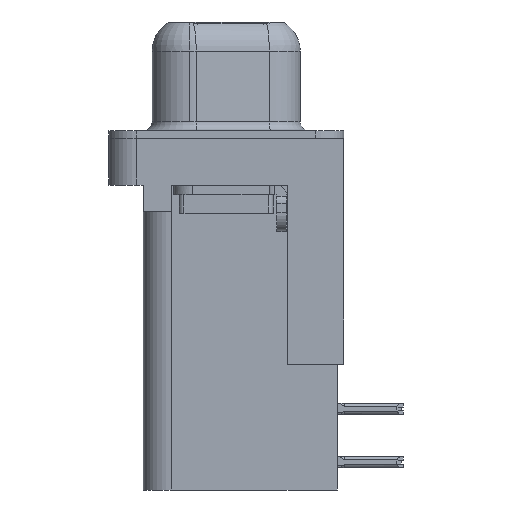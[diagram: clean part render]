
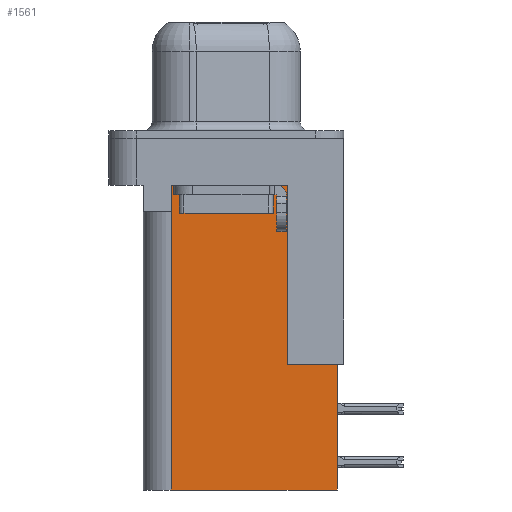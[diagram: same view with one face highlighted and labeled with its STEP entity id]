
A CAD part, left-side view. The second image highlights one B-rep face of the part: STEP entity #1561.
In plain terms, the highlighted planar face has unit normal (-1, 0, 0).
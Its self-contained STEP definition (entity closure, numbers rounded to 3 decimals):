
#509 = CARTESIAN_POINT ( 'NONE',  ( 3.79, 2.925, -18.76 ) ) ;
#693 = CARTESIAN_POINT ( 'NONE',  ( 3.79, 2.895, -3.9 ) ) ;
#821 = CARTESIAN_POINT ( 'NONE',  ( 3.79, 2.895, -3.9 ) ) ;
#904 = VECTOR ( 'NONE', #14009, 1000. ) ;
#1063 = DIRECTION ( 'NONE',  ( 0., 1., 0. ) ) ;
#1561 = ADVANCED_FACE ( 'NONE', ( #11364 ), #18926, .F. ) ;
#1729 = CARTESIAN_POINT ( 'NONE',  ( 3.79, -3.295, -12.05 ) ) ;
#1950 = EDGE_CURVE ( 'NONE', #13787, #18662, #6136, .T. ) ;
#2340 = CARTESIAN_POINT ( 'NONE',  ( 3.79, -3.295, -18.76 ) ) ;
#2726 = CARTESIAN_POINT ( 'NONE',  ( 3.79, -6.295, -12.05 ) ) ;
#2763 = CARTESIAN_POINT ( 'NONE',  ( 3.79, 0., -3.9 ) ) ;
#2947 = ORIENTED_EDGE ( 'NONE', *, *, #11990, .T. ) ;
#3648 = VECTOR ( 'NONE', #15881, 1000. ) ;
#3686 = CARTESIAN_POINT ( 'NONE',  ( 3.79, 2.925, -18.76 ) ) ;
#4226 = VERTEX_POINT ( 'NONE', #11945 ) ;
#4227 = CARTESIAN_POINT ( 'NONE',  ( 3.79, -3.295, -2.5 ) ) ;
#4406 = DIRECTION ( 'NONE',  ( 0., 1., 0. ) ) ;
#4722 = LINE ( 'NONE', #3686, #17510 ) ;
#5367 = DIRECTION ( 'NONE',  ( 0., 0., 1. ) ) ;
#5837 = EDGE_CURVE ( 'NONE', #14403, #13787, #19545, .T. ) ;
#5946 = ORIENTED_EDGE ( 'NONE', *, *, #15339, .T. ) ;
#6136 = LINE ( 'NONE', #2340, #15546 ) ;
#6144 = CARTESIAN_POINT ( 'NONE',  ( 3.79, -3.295, -18.76 ) ) ;
#6197 = LINE ( 'NONE', #2726, #14563 ) ;
#6488 = VERTEX_POINT ( 'NONE', #17413 ) ;
#7244 = ORIENTED_EDGE ( 'NONE', *, *, #15857, .T. ) ;
#7778 = ORIENTED_EDGE ( 'NONE', *, *, #9642, .F. ) ;
#8051 = LINE ( 'NONE', #4227, #3648 ) ;
#8122 = VERTEX_POINT ( 'NONE', #20548 ) ;
#9415 = EDGE_LOOP ( 'NONE', ( #7244, #16502, #11389, #7778, #17585, #16197, #2947, #5946 ) ) ;
#9642 = EDGE_CURVE ( 'NONE', #18662, #8122, #4722, .T. ) ;
#9743 = LINE ( 'NONE', #693, #904 ) ;
#10104 = CARTESIAN_POINT ( 'NONE',  ( 3.79, -5.925, -18.76 ) ) ;
#11345 = DIRECTION ( 'NONE',  ( 0., 0., -1. ) ) ;
#11364 = FACE_OUTER_BOUND ( 'NONE', #9415, .T. ) ;
#11389 = ORIENTED_EDGE ( 'NONE', *, *, #13545, .T. ) ;
#11547 = CARTESIAN_POINT ( 'NONE',  ( 3.79, -3.295, -18.76 ) ) ;
#11945 = CARTESIAN_POINT ( 'NONE',  ( 3.79, 2.895, -2.5 ) ) ;
#11990 = EDGE_CURVE ( 'NONE', #14403, #14978, #6197, .T. ) ;
#12329 = DIRECTION ( 'NONE',  ( 0., 1., 0. ) ) ;
#12849 = EDGE_CURVE ( 'NONE', #4226, #16436, #9743, .T. ) ;
#13545 = EDGE_CURVE ( 'NONE', #16436, #8122, #18074, .T. ) ;
#13787 = VERTEX_POINT ( 'NONE', #10104 ) ;
#14009 = DIRECTION ( 'NONE',  ( 0., 0., -1. ) ) ;
#14403 = VERTEX_POINT ( 'NONE', #17816 ) ;
#14563 = VECTOR ( 'NONE', #1063, 1000. ) ;
#14978 = VERTEX_POINT ( 'NONE', #1729 ) ;
#14981 = DIRECTION ( 'NONE',  ( 0., 1., 0. ) ) ;
#15105 = VECTOR ( 'NONE', #11345, 1000. ) ;
#15339 = EDGE_CURVE ( 'NONE', #14978, #6488, #16418, .T. ) ;
#15546 = VECTOR ( 'NONE', #12329, 1000. ) ;
#15857 = EDGE_CURVE ( 'NONE', #6488, #4226, #8051, .T. ) ;
#15881 = DIRECTION ( 'NONE',  ( 0., 1., 0. ) ) ;
#16197 = ORIENTED_EDGE ( 'NONE', *, *, #5837, .F. ) ;
#16418 = LINE ( 'NONE', #6144, #20874 ) ;
#16436 = VERTEX_POINT ( 'NONE', #821 ) ;
#16502 = ORIENTED_EDGE ( 'NONE', *, *, #12849, .T. ) ;
#17326 = AXIS2_PLACEMENT_3D ( 'NONE', #11547, #17939, #14981 ) ;
#17413 = CARTESIAN_POINT ( 'NONE',  ( 3.79, -3.295, -2.5 ) ) ;
#17510 = VECTOR ( 'NONE', #5367, 1000. ) ;
#17585 = ORIENTED_EDGE ( 'NONE', *, *, #1950, .F. ) ;
#17816 = CARTESIAN_POINT ( 'NONE',  ( 3.79, -5.925, -12.05 ) ) ;
#17939 = DIRECTION ( 'NONE',  ( 1., 0., 0. ) ) ;
#18074 = LINE ( 'NONE', #2763, #21464 ) ;
#18662 = VERTEX_POINT ( 'NONE', #509 ) ;
#18926 = PLANE ( 'NONE',  #17326 ) ;
#19498 = DIRECTION ( 'NONE',  ( 0., 0., 1. ) ) ;
#19545 = LINE ( 'NONE', #21328, #15105 ) ;
#20548 = CARTESIAN_POINT ( 'NONE',  ( 3.79, 2.925, -3.9 ) ) ;
#20874 = VECTOR ( 'NONE', #19498, 1000. ) ;
#21328 = CARTESIAN_POINT ( 'NONE',  ( 3.79, -5.925, -2. ) ) ;
#21464 = VECTOR ( 'NONE', #4406, 1000. ) ;
